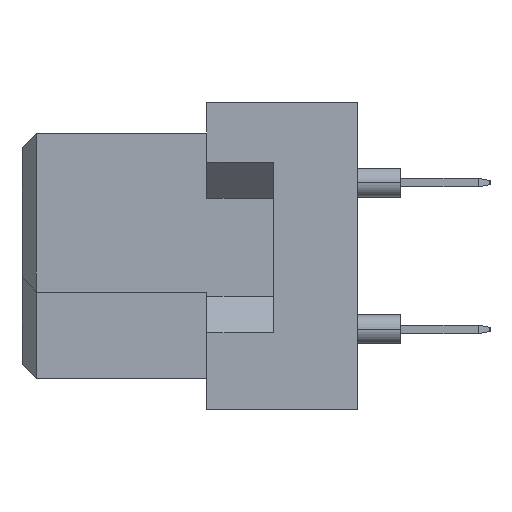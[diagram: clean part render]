
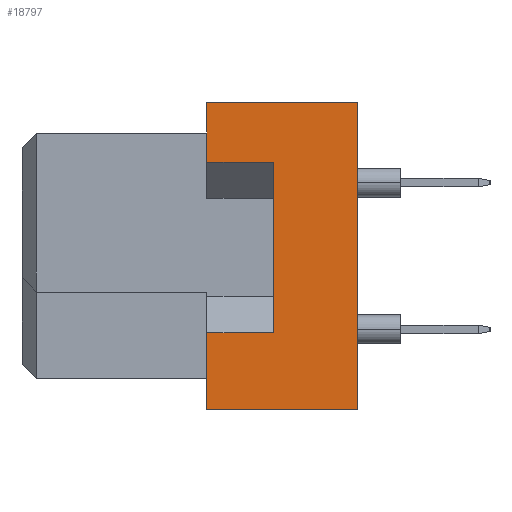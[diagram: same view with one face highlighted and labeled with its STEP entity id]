
A CAD part, left-side view. The second image highlights one B-rep face of the part: STEP entity #18797.
In plain terms, the highlighted planar face has unit normal (-1, 0, 0).
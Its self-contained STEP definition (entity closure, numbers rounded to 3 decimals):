
#308 = DIRECTION ( 'NONE',  ( 0., 1., 0. ) ) ;
#470 = EDGE_CURVE ( 'NONE', #4962, #4666, #5297, .T. ) ;
#691 = VECTOR ( 'NONE', #17564, 1000. ) ;
#951 = DIRECTION ( 'NONE',  ( 0., 0., 1. ) ) ;
#1363 = LINE ( 'NONE', #7868, #6495 ) ;
#1478 = FACE_OUTER_BOUND ( 'NONE', #14174, .T. ) ;
#1914 = VECTOR ( 'NONE', #10696, 1000. ) ;
#1918 = CARTESIAN_POINT ( 'NONE',  ( -27.5, -11.6, 5.3 ) ) ;
#2423 = VECTOR ( 'NONE', #8442, 1000. ) ;
#2454 = CARTESIAN_POINT ( 'NONE',  ( -27.5, -11.6, -5.3 ) ) ;
#2665 = CARTESIAN_POINT ( 'NONE',  ( -27.5, -6.4, -5.3 ) ) ;
#2826 = ORIENTED_EDGE ( 'NONE', *, *, #10714, .F. ) ;
#3095 = CARTESIAN_POINT ( 'NONE',  ( -27.5, -6.4, 5.3 ) ) ;
#3124 = LINE ( 'NONE', #9612, #2423 ) ;
#3431 = VERTEX_POINT ( 'NONE', #9897 ) ;
#4258 = LINE ( 'NONE', #2665, #20829 ) ;
#4360 = DIRECTION ( 'NONE',  ( 0., 1., 0. ) ) ;
#4571 = DIRECTION ( 'NONE',  ( 0., 0., 1. ) ) ;
#4666 = VERTEX_POINT ( 'NONE', #11726 ) ;
#4962 = VERTEX_POINT ( 'NONE', #17571 ) ;
#5077 = DIRECTION ( 'NONE',  ( 0., 0., 1. ) ) ;
#5297 = LINE ( 'NONE', #13255, #12730 ) ;
#5745 = ORIENTED_EDGE ( 'NONE', *, *, #470, .F. ) ;
#5797 = CARTESIAN_POINT ( 'NONE',  ( -27.5, -11.6, 5.3 ) ) ;
#5963 = CARTESIAN_POINT ( 'NONE',  ( -27.5, -8.7, 3.25 ) ) ;
#6150 = ORIENTED_EDGE ( 'NONE', *, *, #6451, .T. ) ;
#6451 = EDGE_CURVE ( 'NONE', #12960, #17032, #16392, .T. ) ;
#6495 = VECTOR ( 'NONE', #10846, 1000. ) ;
#7497 = EDGE_CURVE ( 'NONE', #15350, #12960, #20359, .T. ) ;
#7603 = VECTOR ( 'NONE', #4360, 1000. ) ;
#7668 = VECTOR ( 'NONE', #308, 1000. ) ;
#7678 = PLANE ( 'NONE',  #7893 ) ;
#7679 = LINE ( 'NONE', #2454, #7603 ) ;
#7868 = CARTESIAN_POINT ( 'NONE',  ( -27.5, -8.7, -2.65 ) ) ;
#7893 = AXIS2_PLACEMENT_3D ( 'NONE', #9259, #17657, #4571 ) ;
#8380 = CARTESIAN_POINT ( 'NONE',  ( -27.5, -11.6, -5.3 ) ) ;
#8442 = DIRECTION ( 'NONE',  ( 0., 0., 1. ) ) ;
#9158 = CARTESIAN_POINT ( 'NONE',  ( -27.5, -8.7, 3.25 ) ) ;
#9227 = ORIENTED_EDGE ( 'NONE', *, *, #11497, .F. ) ;
#9259 = CARTESIAN_POINT ( 'NONE',  ( -27.5, -11.6, 5.3 ) ) ;
#9612 = CARTESIAN_POINT ( 'NONE',  ( -27.5, -8.7, -2.65 ) ) ;
#9897 = CARTESIAN_POINT ( 'NONE',  ( -27.5, -6.4, 3.25 ) ) ;
#10696 = DIRECTION ( 'NONE',  ( 0., 0., 1. ) ) ;
#10714 = EDGE_CURVE ( 'NONE', #12137, #3431, #14040, .T. ) ;
#10846 = DIRECTION ( 'NONE',  ( 0., 1., 0. ) ) ;
#11067 = ORIENTED_EDGE ( 'NONE', *, *, #14603, .F. ) ;
#11497 = EDGE_CURVE ( 'NONE', #12662, #12137, #3124, .T. ) ;
#11726 = CARTESIAN_POINT ( 'NONE',  ( -27.5, -6.4, -2.65 ) ) ;
#11788 = ORIENTED_EDGE ( 'NONE', *, *, #17348, .T. ) ;
#12137 = VERTEX_POINT ( 'NONE', #5963 ) ;
#12662 = VERTEX_POINT ( 'NONE', #19402 ) ;
#12730 = VECTOR ( 'NONE', #5077, 1000. ) ;
#12960 = VERTEX_POINT ( 'NONE', #17479 ) ;
#13255 = CARTESIAN_POINT ( 'NONE',  ( -27.5, -6.4, -5.3 ) ) ;
#13876 = ORIENTED_EDGE ( 'NONE', *, *, #7497, .T. ) ;
#14040 = LINE ( 'NONE', #9158, #691 ) ;
#14174 = EDGE_LOOP ( 'NONE', ( #11788, #5745, #17742, #13876, #6150, #11067, #2826, #9227 ) ) ;
#14603 = EDGE_CURVE ( 'NONE', #3431, #17032, #4258, .T. ) ;
#14738 = EDGE_CURVE ( 'NONE', #15350, #4962, #7679, .T. ) ;
#15350 = VERTEX_POINT ( 'NONE', #8380 ) ;
#16392 = LINE ( 'NONE', #1918, #7668 ) ;
#17032 = VERTEX_POINT ( 'NONE', #3095 ) ;
#17348 = EDGE_CURVE ( 'NONE', #12662, #4666, #1363, .T. ) ;
#17479 = CARTESIAN_POINT ( 'NONE',  ( -27.5, -11.6, 5.3 ) ) ;
#17564 = DIRECTION ( 'NONE',  ( 0., 1., 0. ) ) ;
#17571 = CARTESIAN_POINT ( 'NONE',  ( -27.5, -6.4, -5.3 ) ) ;
#17657 = DIRECTION ( 'NONE',  ( -1., 0., 0. ) ) ;
#17742 = ORIENTED_EDGE ( 'NONE', *, *, #14738, .F. ) ;
#18797 = ADVANCED_FACE ( 'NONE', ( #1478 ), #7678, .T. ) ;
#19402 = CARTESIAN_POINT ( 'NONE',  ( -27.5, -8.7, -2.65 ) ) ;
#20359 = LINE ( 'NONE', #5797, #1914 ) ;
#20829 = VECTOR ( 'NONE', #951, 1000. ) ;
